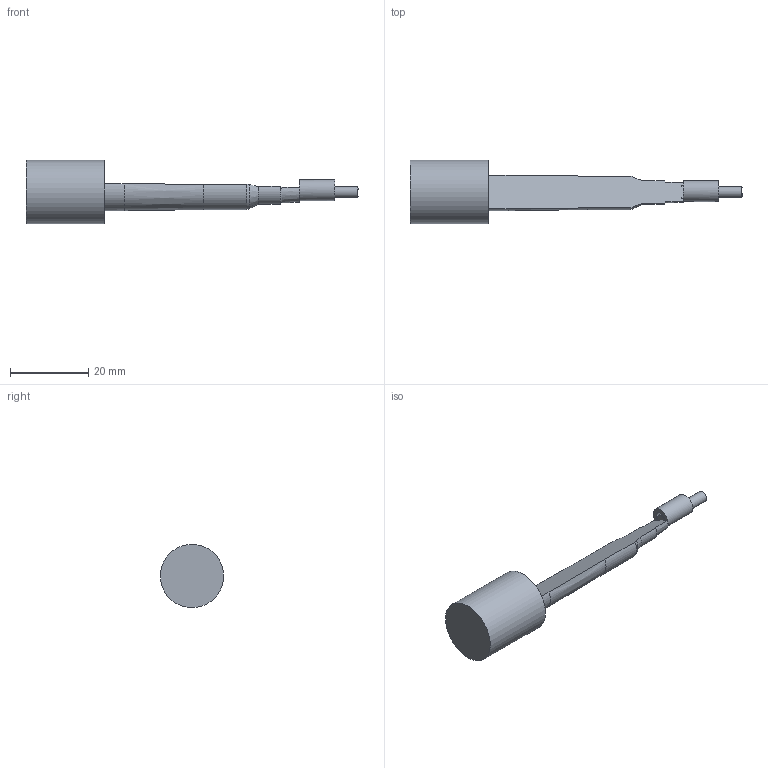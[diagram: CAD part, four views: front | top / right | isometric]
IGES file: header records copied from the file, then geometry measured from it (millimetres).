
Global section: file name: chamber reamer.223 5.56 Assembly; native system: Autodesk Inventor 2019; preprocessor: unknown; author: user; date: 20200917.142330; units: millimetre
Bounding box: 84.85 x 16.15 x 16.17 mm (x, y, z)
Volume: 5774.3 mm3; surface area: 2904 mm2
Topology: 2 solids, 2 shells, 24 faces, 61 edges, 42 vertices
Faces by surface type: bspline 24
